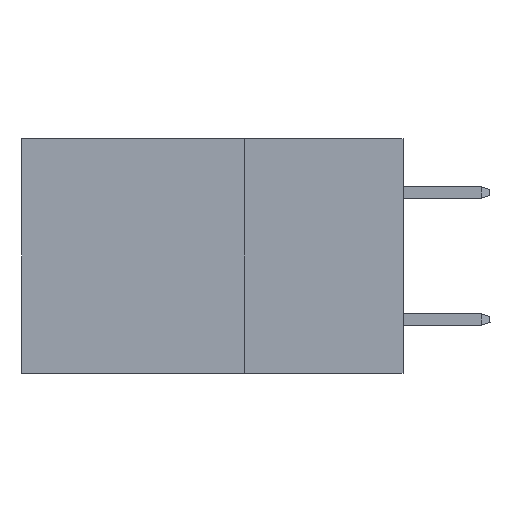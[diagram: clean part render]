
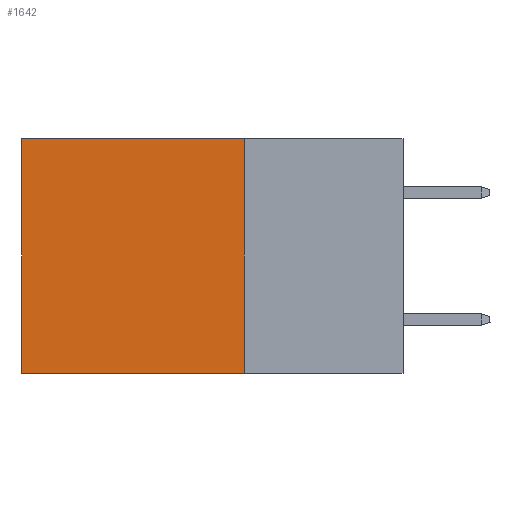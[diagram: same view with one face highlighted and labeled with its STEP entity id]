
A CAD part, left-side view. The second image highlights one B-rep face of the part: STEP entity #1642.
In plain terms, the highlighted planar face has unit normal (-1, 0, 0).
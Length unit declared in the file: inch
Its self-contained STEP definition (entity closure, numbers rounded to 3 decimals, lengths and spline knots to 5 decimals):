
#293 = VECTOR ( 'NONE', #8233, 39.37008 ) ;
#1208 = CARTESIAN_POINT ( 'NONE',  ( 0.2875, 0.25, 0. ) ) ;
#1628 = CARTESIAN_POINT ( 'NONE',  ( 0.2875, 0.6, 0. ) ) ;
#1642 = ADVANCED_FACE ( 'NONE', ( #1787 ), #1858, .F. ) ;
#1787 = FACE_OUTER_BOUND ( 'NONE', #9578, .T. ) ;
#1858 = PLANE ( 'NONE',  #6491 ) ;
#2305 = ORIENTED_EDGE ( 'NONE', *, *, #2376, .T. ) ;
#2376 = EDGE_CURVE ( 'NONE', #8720, #2926, #11332, .T. ) ;
#2695 = ORIENTED_EDGE ( 'NONE', *, *, #8020, .F. ) ;
#2890 = VERTEX_POINT ( 'NONE', #3659 ) ;
#2926 = VERTEX_POINT ( 'NONE', #1628 ) ;
#3382 = CARTESIAN_POINT ( 'NONE',  ( 0.2875, 0.25, -0.37 ) ) ;
#3536 = ORIENTED_EDGE ( 'NONE', *, *, #11778, .F. ) ;
#3659 = CARTESIAN_POINT ( 'NONE',  ( 0.2875, 0.6, -0.37 ) ) ;
#3718 = LINE ( 'NONE', #11689, #7487 ) ;
#4030 = DIRECTION ( 'NONE',  ( 1., 0., 0. ) ) ;
#4276 = DIRECTION ( 'NONE',  ( 0., 0., -1. ) ) ;
#4563 = VERTEX_POINT ( 'NONE', #3382 ) ;
#4642 = DIRECTION ( 'NONE',  ( 0., 1., 0. ) ) ;
#5384 = CARTESIAN_POINT ( 'NONE',  ( 0.2875, 0.25, 0. ) ) ;
#5403 = EDGE_CURVE ( 'NONE', #2926, #2890, #8302, .T. ) ;
#5744 = LINE ( 'NONE', #11677, #6799 ) ;
#5794 = CARTESIAN_POINT ( 'NONE',  ( 0.2875, 0.25, 0. ) ) ;
#5865 = DIRECTION ( 'NONE',  ( 0., 0., -1. ) ) ;
#6491 = AXIS2_PLACEMENT_3D ( 'NONE', #5794, #4030, #5865 ) ;
#6737 = DIRECTION ( 'NONE',  ( 0., 0., -1. ) ) ;
#6799 = VECTOR ( 'NONE', #4642, 39.37008 ) ;
#7206 = CARTESIAN_POINT ( 'NONE',  ( 0.2875, 0.6, 0. ) ) ;
#7487 = VECTOR ( 'NONE', #6737, 39.37008 ) ;
#8020 = EDGE_CURVE ( 'NONE', #4563, #2890, #5744, .T. ) ;
#8233 = DIRECTION ( 'NONE',  ( 0., 1., 0. ) ) ;
#8302 = LINE ( 'NONE', #7206, #9637 ) ;
#8373 = ORIENTED_EDGE ( 'NONE', *, *, #5403, .T. ) ;
#8720 = VERTEX_POINT ( 'NONE', #1208 ) ;
#9578 = EDGE_LOOP ( 'NONE', ( #8373, #2695, #3536, #2305 ) ) ;
#9637 = VECTOR ( 'NONE', #4276, 39.37008 ) ;
#11332 = LINE ( 'NONE', #5384, #293 ) ;
#11677 = CARTESIAN_POINT ( 'NONE',  ( 0.2875, 0.25, -0.37 ) ) ;
#11689 = CARTESIAN_POINT ( 'NONE',  ( 0.2875, 0.25, 0. ) ) ;
#11778 = EDGE_CURVE ( 'NONE', #8720, #4563, #3718, .T. ) ;
